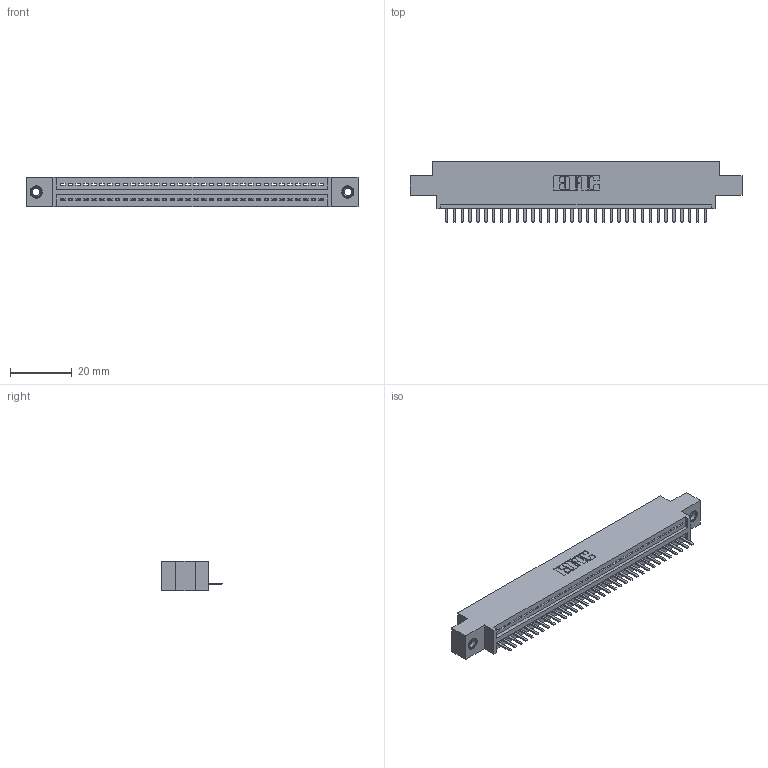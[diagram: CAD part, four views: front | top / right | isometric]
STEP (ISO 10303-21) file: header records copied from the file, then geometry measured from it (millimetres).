
FILE_DESCRIPTION (( 'STEP AP203' ), '1' );
FILE_NAME ('345-034-520-607.STEP', '2019-10-07T18:33:21', ( '' ), ( '' ), 'SwSTEP 2.0', 'SolidWorks 2016', '' );
FILE_SCHEMA (( 'CONFIG_CONTROL_DESIGN' ));
Length unit declared in the file: inch
Products named in the file (4): 345 Part_0.170 Offset - 0.156 Dia-TI; 345-292-001_345-293-120; 345-034-520-607; 345-250-001_345-250-005-103
Assembly tree (37 placements, depth 2):
  345-034-520-607
    345 Part_0.170 Offset - 0.156 Dia-TI
    345-292-001_345-293-120  x34
    345-250-001_345-250-005-103  x2
Bounding box: 107.57 x 19.68 x 9.4 mm (x, y, z)
Volume: 9926.8 mm3; surface area: 12922.2 mm2
Topology: 37 solids, 37 shells, 2298 faces, 6745 edges, 4398 vertices
Faces by surface type: plane 1544, cylinder 738, cone 12, torus 4
Entity records: 28098 total; most frequent: CARTESIAN_POINT 4861, ORIENTED_EDGE 4810, DIRECTION 4271, EDGE_CURVE 2405, LINE 2113, VECTOR 2113, VERTEX_POINT 1596, AXIS2_PLACEMENT_3D 1079
